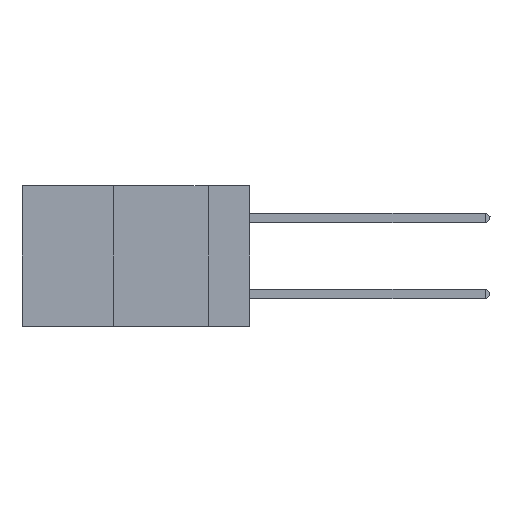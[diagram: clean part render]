
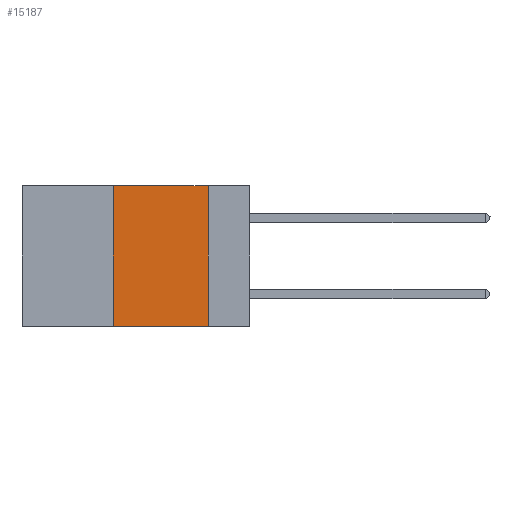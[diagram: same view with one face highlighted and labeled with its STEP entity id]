
A CAD part, left-side view. The second image highlights one B-rep face of the part: STEP entity #15187.
In plain terms, the highlighted planar face has unit normal (-1, 0, 0).
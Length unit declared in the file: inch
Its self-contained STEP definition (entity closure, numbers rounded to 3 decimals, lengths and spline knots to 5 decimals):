
#45 = CARTESIAN_POINT ( 'NONE',  ( 0., 0.36, -0.37 ) ) ;
#55 = DIRECTION ( 'NONE',  ( 0., 0., -1. ) ) ;
#958 = VECTOR ( 'NONE', #9105, 39.37008 ) ;
#1072 = EDGE_CURVE ( 'NONE', #5311, #4610, #2130, .T. ) ;
#1752 = AXIS2_PLACEMENT_3D ( 'NONE', #6176, #5944, #55 ) ;
#1952 = LINE ( 'NONE', #12202, #2446 ) ;
#2130 = LINE ( 'NONE', #6960, #15771 ) ;
#2301 = VERTEX_POINT ( 'NONE', #2959 ) ;
#2446 = VECTOR ( 'NONE', #14158, 39.37008 ) ;
#2781 = ORIENTED_EDGE ( 'NONE', *, *, #4218, .F. ) ;
#2944 = EDGE_CURVE ( 'NONE', #5311, #18084, #10158, .T. ) ;
#2959 = CARTESIAN_POINT ( 'NONE',  ( 0., 0.11, 0. ) ) ;
#4218 = EDGE_CURVE ( 'NONE', #2301, #18084, #23527, .T. ) ;
#4610 = VERTEX_POINT ( 'NONE', #21824 ) ;
#5311 = VERTEX_POINT ( 'NONE', #45 ) ;
#5541 = EDGE_CURVE ( 'NONE', #4610, #2301, #1952, .T. ) ;
#5944 = DIRECTION ( 'NONE',  ( 1., 0., 0. ) ) ;
#6004 = ORIENTED_EDGE ( 'NONE', *, *, #5541, .F. ) ;
#6176 = CARTESIAN_POINT ( 'NONE',  ( 0., 0.6, 0. ) ) ;
#6825 = VECTOR ( 'NONE', #9860, 39.37008 ) ;
#6887 = ORIENTED_EDGE ( 'NONE', *, *, #2944, .T. ) ;
#6960 = CARTESIAN_POINT ( 'NONE',  ( 0., 0.36, 0. ) ) ;
#7124 = DIRECTION ( 'NONE',  ( 0., 0., 1. ) ) ;
#7828 = CARTESIAN_POINT ( 'NONE',  ( 0., 0.6, -0.37 ) ) ;
#7918 = ORIENTED_EDGE ( 'NONE', *, *, #1072, .F. ) ;
#9105 = DIRECTION ( 'NONE',  ( 0., 0., -1. ) ) ;
#9860 = DIRECTION ( 'NONE',  ( 0., -1., 0. ) ) ;
#10158 = LINE ( 'NONE', #7828, #6825 ) ;
#11888 = PLANE ( 'NONE',  #1752 ) ;
#12131 = EDGE_LOOP ( 'NONE', ( #2781, #6004, #7918, #6887 ) ) ;
#12202 = CARTESIAN_POINT ( 'NONE',  ( 0., 0.6, 0. ) ) ;
#14158 = DIRECTION ( 'NONE',  ( 0., -1., 0. ) ) ;
#15187 = ADVANCED_FACE ( 'NONE', ( #15933 ), #11888, .F. ) ;
#15771 = VECTOR ( 'NONE', #7124, 39.37008 ) ;
#15933 = FACE_OUTER_BOUND ( 'NONE', #12131, .T. ) ;
#16403 = CARTESIAN_POINT ( 'NONE',  ( 0., 0.11, -0.37 ) ) ;
#18084 = VERTEX_POINT ( 'NONE', #16403 ) ;
#21824 = CARTESIAN_POINT ( 'NONE',  ( 0., 0.36, 0. ) ) ;
#21929 = CARTESIAN_POINT ( 'NONE',  ( 0., 0.11, 0. ) ) ;
#23527 = LINE ( 'NONE', #21929, #958 ) ;
